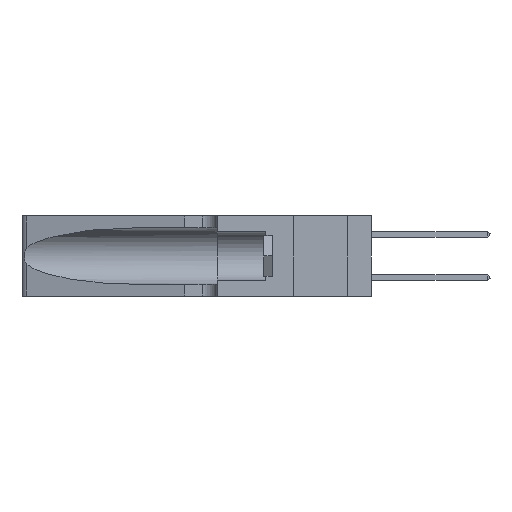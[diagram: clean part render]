
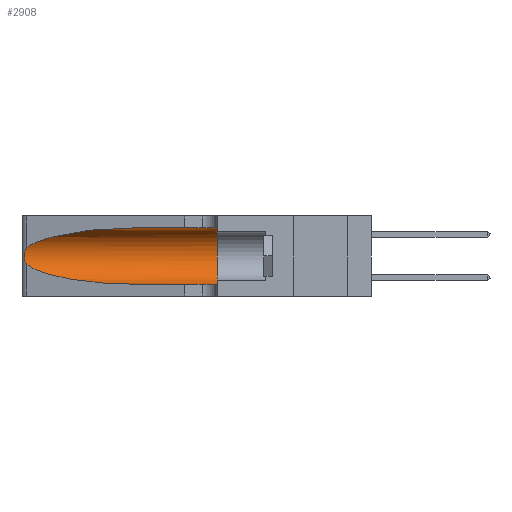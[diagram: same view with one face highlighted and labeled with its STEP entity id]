
A CAD part, left-side view. The second image highlights one B-rep face of the part: STEP entity #2908.
In plain terms, the highlighted cylindrical face has radius 3.308 mm (diameter 6.617 mm), a partial arc.
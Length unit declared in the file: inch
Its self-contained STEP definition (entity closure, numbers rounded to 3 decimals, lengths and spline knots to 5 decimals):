
#366 = LINE ( 'NONE', #45473, #38347 ) ;
#631 = AXIS2_PLACEMENT_3D ( 'NONE', #20286, #46024, #23983 ) ;
#1108 = CIRCLE ( 'NONE', #631, 0.13025 ) ;
#1245 = CARTESIAN_POINT ( 'NONE',  ( 0.25487, 1.22718, 0.14631 ) ) ;
#2223 = AXIS2_PLACEMENT_3D ( 'NONE', #18483, #44234, #40565 ) ;
#2688 =( BOUNDED_CURVE ( )  B_SPLINE_CURVE ( 3, ( #45576, #19834, #27256, #5217 ),
 .UNSPECIFIED., .F., .T. ) 
 B_SPLINE_CURVE_WITH_KNOTS ( ( 4, 4 ),
 ( 3.44316, 4.71239 ),
 .UNSPECIFIED. ) 
 CURVE ( )  GEOMETRIC_REPRESENTATION_ITEM ( )  RATIONAL_B_SPLINE_CURVE ( ( 1., 0.87, 0.87, 1. ) ) 
 REPRESENTATION_ITEM ( '' )  );
#2908 = ADVANCED_FACE ( 'NONE', ( #26546 ), #42681, .F. ) ;
#2981 = CARTESIAN_POINT ( 'NONE',  ( 0.1305, 1.61858, 0.05475 ) ) ;
#3070 = CARTESIAN_POINT ( 'NONE',  ( 0.26075, 1.23896, 0.178 ) ) ;
#3170 = CARTESIAN_POINT ( 'NONE',  ( 0.1305, 0.35, 0.05475 ) ) ;
#5217 = CARTESIAN_POINT ( 'NONE',  ( 0.1305, 0.72297, 0.05475 ) ) ;
#5929 = ORIENTED_EDGE ( 'NONE', *, *, #32463, .T. ) ;
#6749 = CARTESIAN_POINT ( 'NONE',  ( 0.25856, 1.23593, 0.16098 ) ) ;
#8244 = ORIENTED_EDGE ( 'NONE', *, *, #46814, .F. ) ;
#9110 = VERTEX_POINT ( 'NONE', #12089 ) ;
#10427 = CARTESIAN_POINT ( 'NONE',  ( 0.25639, 1.23186, 0.15144 ) ) ;
#11200 = B_SPLINE_CURVE_WITH_KNOTS ( 'NONE', 3,
 ( #39710, #13957, #35995, #43427, #21351, #47092, #25084, #3070, #28789, #6749, #32472, #10427, #36152, #14111 ),
 .UNSPECIFIED., .F., .F.,
 ( 4, 2, 2, 2, 2, 2, 4 ),
 ( 0., 0.00027, 0.00053, 0.00107, 0.0016, 0.00187, 0.00214 ),
 .UNSPECIFIED. ) ;
#11224 = CARTESIAN_POINT ( 'NONE',  ( 0.25487, 1.22718, 0.22369 ) ) ;
#12089 = CARTESIAN_POINT ( 'NONE',  ( 0.1305, 0.72297, 0.31525 ) ) ;
#13905 = ORIENTED_EDGE ( 'NONE', *, *, #33196, .T. ) ;
#13957 = CARTESIAN_POINT ( 'NONE',  ( 0.25555, 1.22994, 0.2215 ) ) ;
#14111 = CARTESIAN_POINT ( 'NONE',  ( 0.25487, 1.22718, 0.14631 ) ) ;
#14283 = CARTESIAN_POINT ( 'NONE',  ( 0.1305, 0.72297, 0.31525 ) ) ;
#16585 = VERTEX_POINT ( 'NONE', #37742 ) ;
#17995 = CARTESIAN_POINT ( 'NONE',  ( 0.2373, 1.15595, 0.28018 ) ) ;
#18483 = CARTESIAN_POINT ( 'NONE',  ( 0.1305, 1.61858, 0.185 ) ) ;
#19403 = EDGE_CURVE ( 'NONE', #19573, #37965, #11200, .T. ) ;
#19573 = VERTEX_POINT ( 'NONE', #11224 ) ;
#19621 = VECTOR ( 'NONE', #36063, 39.37008 ) ;
#19725 = DIRECTION ( 'NONE',  ( 0., -1., 0. ) ) ;
#19834 = CARTESIAN_POINT ( 'NONE',  ( 0.2373, 1.15595, 0.08982 ) ) ;
#20286 = CARTESIAN_POINT ( 'NONE',  ( 0.1305, 0.35, 0.185 ) ) ;
#20444 = EDGE_CURVE ( 'NONE', #37965, #40035, #2688, .T. ) ;
#21351 = CARTESIAN_POINT ( 'NONE',  ( 0.25854, 1.2359, 0.20912 ) ) ;
#23983 = DIRECTION ( 'NONE',  ( 0., 0., 1. ) ) ;
#24042 = CARTESIAN_POINT ( 'NONE',  ( 0.1305, 0.72297, 0.05475 ) ) ;
#24778 =( BOUNDED_CURVE ( )  B_SPLINE_CURVE ( 3, ( #14283, #40053, #17995, #43758 ),
 .UNSPECIFIED., .F., .F. ) 
 B_SPLINE_CURVE_WITH_KNOTS ( ( 4, 4 ),
 ( 1.5708, 2.84003 ),
 .UNSPECIFIED. ) 
 CURVE ( )  GEOMETRIC_REPRESENTATION_ITEM ( )  RATIONAL_B_SPLINE_CURVE ( ( 1., 0.87, 0.87, 1. ) ) 
 REPRESENTATION_ITEM ( '' )  );
#25084 = CARTESIAN_POINT ( 'NONE',  ( 0.26075, 1.23896, 0.19203 ) ) ;
#26546 = FACE_OUTER_BOUND ( 'NONE', #46596, .T. ) ;
#27256 = CARTESIAN_POINT ( 'NONE',  ( 0.18966, 0.96281, 0.05475 ) ) ;
#28789 = CARTESIAN_POINT ( 'NONE',  ( 0.26017, 1.23833, 0.17102 ) ) ;
#30125 = ORIENTED_EDGE ( 'NONE', *, *, #43050, .F. ) ;
#30629 = LINE ( 'NONE', #2981, #19621 ) ;
#30686 = ORIENTED_EDGE ( 'NONE', *, *, #20444, .T. ) ;
#32463 = EDGE_CURVE ( 'NONE', #40035, #41474, #30629, .T. ) ;
#32472 = CARTESIAN_POINT ( 'NONE',  ( 0.25789, 1.23486, 0.15765 ) ) ;
#33196 = EDGE_CURVE ( 'NONE', #9110, #19573, #24778, .T. ) ;
#35995 = CARTESIAN_POINT ( 'NONE',  ( 0.25639, 1.23184, 0.21858 ) ) ;
#36063 = DIRECTION ( 'NONE',  ( 0., -1., 0. ) ) ;
#36152 = CARTESIAN_POINT ( 'NONE',  ( 0.25555, 1.22993, 0.14849 ) ) ;
#37742 = CARTESIAN_POINT ( 'NONE',  ( 0.1305, 0.35, 0.31525 ) ) ;
#37965 = VERTEX_POINT ( 'NONE', #1245 ) ;
#38347 = VECTOR ( 'NONE', #19725, 39.37008 ) ;
#39710 = CARTESIAN_POINT ( 'NONE',  ( 0.25487, 1.22718, 0.22369 ) ) ;
#40035 = VERTEX_POINT ( 'NONE', #24042 ) ;
#40053 = CARTESIAN_POINT ( 'NONE',  ( 0.18966, 0.96281, 0.31525 ) ) ;
#40565 = DIRECTION ( 'NONE',  ( 0., 0., -1. ) ) ;
#41474 = VERTEX_POINT ( 'NONE', #3170 ) ;
#42681 = CYLINDRICAL_SURFACE ( 'NONE', #2223, 0.13025 ) ;
#43050 = EDGE_CURVE ( 'NONE', #9110, #16585, #366, .T. ) ;
#43427 = CARTESIAN_POINT ( 'NONE',  ( 0.25787, 1.23484, 0.2124 ) ) ;
#43758 = CARTESIAN_POINT ( 'NONE',  ( 0.25487, 1.22718, 0.22369 ) ) ;
#44234 = DIRECTION ( 'NONE',  ( 0., -1., 0. ) ) ;
#45473 = CARTESIAN_POINT ( 'NONE',  ( 0.1305, 1.61858, 0.31525 ) ) ;
#45576 = CARTESIAN_POINT ( 'NONE',  ( 0.25487, 1.22718, 0.14631 ) ) ;
#45600 = ORIENTED_EDGE ( 'NONE', *, *, #19403, .T. ) ;
#46024 = DIRECTION ( 'NONE',  ( 0., 1., 0. ) ) ;
#46596 = EDGE_LOOP ( 'NONE', ( #13905, #45600, #30686, #5929, #8244, #30125 ) ) ;
#46814 = EDGE_CURVE ( 'NONE', #16585, #41474, #1108, .T. ) ;
#47092 = CARTESIAN_POINT ( 'NONE',  ( 0.26018, 1.23835, 0.19895 ) ) ;
